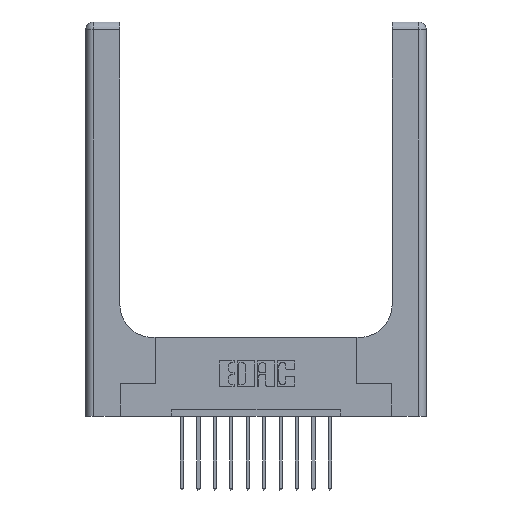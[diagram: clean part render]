
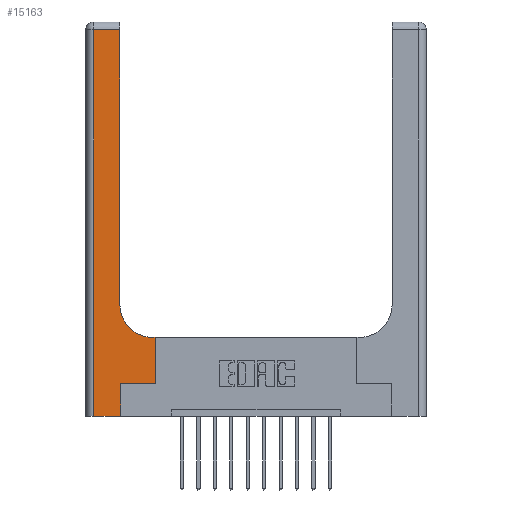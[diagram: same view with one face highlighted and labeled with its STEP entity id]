
A CAD part, top view. The second image highlights one B-rep face of the part: STEP entity #15163.
In plain terms, the highlighted planar face has unit normal (0, 0, 1).
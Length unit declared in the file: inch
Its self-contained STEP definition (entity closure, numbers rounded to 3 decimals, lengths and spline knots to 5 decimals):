
#395 = LINE ( 'NONE', #15587, #14430 ) ;
#480 = ORIENTED_EDGE ( 'NONE', *, *, #5970, .T. ) ;
#729 = CARTESIAN_POINT ( 'NONE',  ( 0.06, 0., 0.37 ) ) ;
#778 = ORIENTED_EDGE ( 'NONE', *, *, #8254, .T. ) ;
#920 = ORIENTED_EDGE ( 'NONE', *, *, #8738, .T. ) ;
#1225 = CARTESIAN_POINT ( 'NONE',  ( 0.265, 0.25, 0.37 ) ) ;
#1920 = EDGE_CURVE ( 'NONE', #16146, #9996, #7978, .T. ) ;
#1956 = ORIENTED_EDGE ( 'NONE', *, *, #8427, .T. ) ;
#2043 = CARTESIAN_POINT ( 'NONE',  ( 0.26, 0.6, 0.37 ) ) ;
#2124 = DIRECTION ( 'NONE',  ( 0., 0., -1. ) ) ;
#2588 = DIRECTION ( 'NONE',  ( 0., 1., 0. ) ) ;
#2852 = CARTESIAN_POINT ( 'NONE',  ( 0.06, 2.94, 0.37 ) ) ;
#2983 = DIRECTION ( 'NONE',  ( 1., 0., 0. ) ) ;
#3101 = EDGE_CURVE ( 'NONE', #11240, #5608, #10677, .T. ) ;
#3791 = ORIENTED_EDGE ( 'NONE', *, *, #1920, .T. ) ;
#3860 = CARTESIAN_POINT ( 'NONE',  ( 0.26, 3., 0.37 ) ) ;
#3972 = ORIENTED_EDGE ( 'NONE', *, *, #3101, .T. ) ;
#4377 = AXIS2_PLACEMENT_3D ( 'NONE', #14400, #13095, #2983 ) ;
#4466 = LINE ( 'NONE', #2043, #15179 ) ;
#4492 = DIRECTION ( 'NONE',  ( 0., -1., 0. ) ) ;
#5086 = LINE ( 'NONE', #3860, #11846 ) ;
#5144 = CARTESIAN_POINT ( 'NONE',  ( 0., 0., 0.37 ) ) ;
#5211 = ORIENTED_EDGE ( 'NONE', *, *, #5612, .T. ) ;
#5237 = VECTOR ( 'NONE', #11975, 39.37008 ) ;
#5608 = VERTEX_POINT ( 'NONE', #8732 ) ;
#5610 = LINE ( 'NONE', #6934, #5237 ) ;
#5612 = EDGE_CURVE ( 'NONE', #11237, #16146, #12383, .T. ) ;
#5722 = CARTESIAN_POINT ( 'NONE',  ( 0.528, 0.6, 0.37 ) ) ;
#5970 = EDGE_CURVE ( 'NONE', #15483, #10126, #5610, .T. ) ;
#5977 = VERTEX_POINT ( 'NONE', #729 ) ;
#6424 = AXIS2_PLACEMENT_3D ( 'NONE', #8500, #2124, #8424 ) ;
#6595 = VERTEX_POINT ( 'NONE', #5722 ) ;
#6934 = CARTESIAN_POINT ( 'NONE',  ( 0., 2.94, 0.37 ) ) ;
#6968 = VECTOR ( 'NONE', #10294, 39.37008 ) ;
#7047 = VECTOR ( 'NONE', #11771, 39.37008 ) ;
#7193 = VECTOR ( 'NONE', #4492, 39.37008 ) ;
#7905 = DIRECTION ( 'NONE',  ( 0., 1., 0. ) ) ;
#7978 = LINE ( 'NONE', #1225, #7047 ) ;
#8254 = EDGE_CURVE ( 'NONE', #6595, #11240, #4466, .T. ) ;
#8424 = DIRECTION ( 'NONE',  ( -1., 0., 0. ) ) ;
#8427 = EDGE_CURVE ( 'NONE', #9996, #6595, #395, .T. ) ;
#8500 = CARTESIAN_POINT ( 'NONE',  ( 0., 3., 0.37 ) ) ;
#8732 = CARTESIAN_POINT ( 'NONE',  ( 0.26, 0.85, 0.37 ) ) ;
#8738 = EDGE_CURVE ( 'NONE', #5608, #15483, #5086, .T. ) ;
#8995 = CARTESIAN_POINT ( 'NONE',  ( 0.265, 0.25, 0.37 ) ) ;
#9636 = PLANE ( 'NONE',  #6424 ) ;
#9996 = VERTEX_POINT ( 'NONE', #12262 ) ;
#10126 = VERTEX_POINT ( 'NONE', #2852 ) ;
#10294 = DIRECTION ( 'NONE',  ( 1., 0., 0. ) ) ;
#10677 = CIRCLE ( 'NONE', #4377, 0.25 ) ;
#10785 = CARTESIAN_POINT ( 'NONE',  ( 0.26, 2.94, 0.37 ) ) ;
#11237 = VERTEX_POINT ( 'NONE', #12192 ) ;
#11240 = VERTEX_POINT ( 'NONE', #12036 ) ;
#11650 = LINE ( 'NONE', #5144, #6968 ) ;
#11771 = DIRECTION ( 'NONE',  ( 1., 0., 0. ) ) ;
#11846 = VECTOR ( 'NONE', #13731, 39.37008 ) ;
#11975 = DIRECTION ( 'NONE',  ( -1., 0., 0. ) ) ;
#12036 = CARTESIAN_POINT ( 'NONE',  ( 0.51, 0.6, 0.37 ) ) ;
#12131 = DIRECTION ( 'NONE',  ( -1., 0., 0. ) ) ;
#12192 = CARTESIAN_POINT ( 'NONE',  ( 0.265, 0., 0.37 ) ) ;
#12262 = CARTESIAN_POINT ( 'NONE',  ( 0.528, 0.25, 0.37 ) ) ;
#12383 = LINE ( 'NONE', #16023, #15953 ) ;
#13095 = DIRECTION ( 'NONE',  ( 0., 0., -1. ) ) ;
#13133 = ORIENTED_EDGE ( 'NONE', *, *, #16138, .T. ) ;
#13731 = DIRECTION ( 'NONE',  ( 0., 1., 0. ) ) ;
#14272 = CARTESIAN_POINT ( 'NONE',  ( 0.06, 3., 0.37 ) ) ;
#14400 = CARTESIAN_POINT ( 'NONE',  ( 0.51, 0.85, 0.37 ) ) ;
#14430 = VECTOR ( 'NONE', #7905, 39.37008 ) ;
#14456 = EDGE_LOOP ( 'NONE', ( #920, #480, #15522, #13133, #5211, #3791, #1956, #778, #3972 ) ) ;
#14641 = EDGE_CURVE ( 'NONE', #10126, #5977, #15720, .T. ) ;
#15163 = ADVANCED_FACE ( 'NONE', ( #15936 ), #9636, .F. ) ;
#15179 = VECTOR ( 'NONE', #12131, 39.37008 ) ;
#15483 = VERTEX_POINT ( 'NONE', #10785 ) ;
#15522 = ORIENTED_EDGE ( 'NONE', *, *, #14641, .T. ) ;
#15587 = CARTESIAN_POINT ( 'NONE',  ( 0.528, 0.25, 0.37 ) ) ;
#15720 = LINE ( 'NONE', #14272, #7193 ) ;
#15936 = FACE_OUTER_BOUND ( 'NONE', #14456, .T. ) ;
#15953 = VECTOR ( 'NONE', #2588, 39.37008 ) ;
#16023 = CARTESIAN_POINT ( 'NONE',  ( 0.265, 0., 0.37 ) ) ;
#16138 = EDGE_CURVE ( 'NONE', #5977, #11237, #11650, .T. ) ;
#16146 = VERTEX_POINT ( 'NONE', #8995 ) ;
